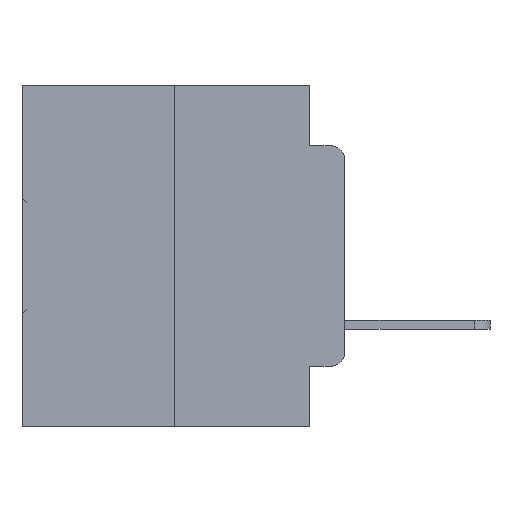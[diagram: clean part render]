
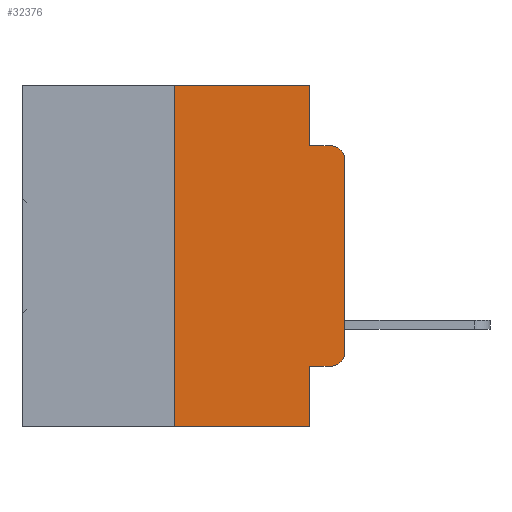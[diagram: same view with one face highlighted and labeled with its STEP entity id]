
A CAD part, left-side view. The second image highlights one B-rep face of the part: STEP entity #32376.
In plain terms, the highlighted planar face has unit normal (-1, 0, 0).
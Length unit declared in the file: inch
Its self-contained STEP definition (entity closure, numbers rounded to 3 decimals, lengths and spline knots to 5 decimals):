
#110 = LINE ( 'NONE', #14499, #1008 ) ;
#382 = ORIENTED_EDGE ( 'NONE', *, *, #10923, .F. ) ;
#1008 = VECTOR ( 'NONE', #17127, 39.37008 ) ;
#1029 = DIRECTION ( 'NONE',  ( 0., -1., 0. ) ) ;
#1550 = CARTESIAN_POINT ( 'NONE',  ( 0., 0.051, 0. ) ) ;
#2625 = EDGE_CURVE ( 'NONE', #13535, #3771, #27099, .T. ) ;
#3015 = ORIENTED_EDGE ( 'NONE', *, *, #16849, .T. ) ;
#3771 = VERTEX_POINT ( 'NONE', #13860 ) ;
#3918 = CIRCLE ( 'NONE', #6936, 0.02 ) ;
#4028 = CARTESIAN_POINT ( 'NONE',  ( 0., 0.051, -0.4115 ) ) ;
#4211 = ORIENTED_EDGE ( 'NONE', *, *, #32056, .T. ) ;
#4632 = CARTESIAN_POINT ( 'NONE',  ( 0., 0.02, -0.3915 ) ) ;
#4680 = VERTEX_POINT ( 'NONE', #14831 ) ;
#5971 = DIRECTION ( 'NONE',  ( 0., 0., 1. ) ) ;
#6571 = CARTESIAN_POINT ( 'NONE',  ( 0., 0.473, 0. ) ) ;
#6590 = VERTEX_POINT ( 'NONE', #17049 ) ;
#6855 = EDGE_CURVE ( 'NONE', #9072, #18997, #19088, .T. ) ;
#6936 = AXIS2_PLACEMENT_3D ( 'NONE', #8356, #26353, #11030 ) ;
#7073 = VERTEX_POINT ( 'NONE', #15179 ) ;
#7368 = DIRECTION ( 'NONE',  ( 0., 0., -1. ) ) ;
#8356 = CARTESIAN_POINT ( 'NONE',  ( 0., 0.02, -0.1085 ) ) ;
#8555 = CARTESIAN_POINT ( 'NONE',  ( 0., 0.25, 0. ) ) ;
#9072 = VERTEX_POINT ( 'NONE', #4028 ) ;
#9272 = DIRECTION ( 'NONE',  ( 0., 0., -1. ) ) ;
#9287 = LINE ( 'NONE', #19518, #15393 ) ;
#10336 = CARTESIAN_POINT ( 'NONE',  ( 0., 0.02, -0.4115 ) ) ;
#10457 = EDGE_CURVE ( 'NONE', #9072, #12935, #26329, .T. ) ;
#10923 = EDGE_CURVE ( 'NONE', #7073, #6590, #9287, .T. ) ;
#10950 = ORIENTED_EDGE ( 'NONE', *, *, #10457, .F. ) ;
#11030 = DIRECTION ( 'NONE',  ( 0., 0., -1. ) ) ;
#11318 = CARTESIAN_POINT ( 'NONE',  ( 0., 0.02, -0.0885 ) ) ;
#11800 = PLANE ( 'NONE',  #18601 ) ;
#12728 = VECTOR ( 'NONE', #21483, 39.37008 ) ;
#12793 = VECTOR ( 'NONE', #22069, 39.37008 ) ;
#12929 = ORIENTED_EDGE ( 'NONE', *, *, #24236, .F. ) ;
#12935 = VERTEX_POINT ( 'NONE', #26229 ) ;
#13535 = VERTEX_POINT ( 'NONE', #28620 ) ;
#13860 = CARTESIAN_POINT ( 'NONE',  ( 0., 0., -0.1085 ) ) ;
#14499 = CARTESIAN_POINT ( 'NONE',  ( 0., 0.051, -0.0885 ) ) ;
#14705 = VERTEX_POINT ( 'NONE', #27469 ) ;
#14831 = CARTESIAN_POINT ( 'NONE',  ( 0., 0.25, -0.5 ) ) ;
#15037 = CIRCLE ( 'NONE', #16231, 0.02 ) ;
#15179 = CARTESIAN_POINT ( 'NONE',  ( 0., 0.25, 0. ) ) ;
#15393 = VECTOR ( 'NONE', #1029, 39.37008 ) ;
#16231 = AXIS2_PLACEMENT_3D ( 'NONE', #4632, #22925, #7368 ) ;
#16281 = CARTESIAN_POINT ( 'NONE',  ( 0., 0.051, -0.4115 ) ) ;
#16462 = DIRECTION ( 'NONE',  ( 0., 0., -1. ) ) ;
#16849 = EDGE_CURVE ( 'NONE', #4680, #12935, #26413, .T. ) ;
#17049 = CARTESIAN_POINT ( 'NONE',  ( 0., 0.051, 0. ) ) ;
#17127 = DIRECTION ( 'NONE',  ( 0., -1., 0. ) ) ;
#17421 = EDGE_CURVE ( 'NONE', #4680, #7073, #21299, .T. ) ;
#17423 = ORIENTED_EDGE ( 'NONE', *, *, #2625, .T. ) ;
#18231 = ORIENTED_EDGE ( 'NONE', *, *, #30620, .F. ) ;
#18601 = AXIS2_PLACEMENT_3D ( 'NONE', #6571, #24701, #9272 ) ;
#18838 = VECTOR ( 'NONE', #27514, 39.37008 ) ;
#18997 = VERTEX_POINT ( 'NONE', #10336 ) ;
#19088 = LINE ( 'NONE', #16281, #25785 ) ;
#19518 = CARTESIAN_POINT ( 'NONE',  ( 0., 0.473, 0. ) ) ;
#19535 = CARTESIAN_POINT ( 'NONE',  ( 0., 0.473, -0.5 ) ) ;
#20516 = VECTOR ( 'NONE', #5971, 39.37008 ) ;
#21299 = LINE ( 'NONE', #8555, #20516 ) ;
#21483 = DIRECTION ( 'NONE',  ( 0., 0., 1. ) ) ;
#22069 = DIRECTION ( 'NONE',  ( 0., -1., 0. ) ) ;
#22751 = VERTEX_POINT ( 'NONE', #11318 ) ;
#22925 = DIRECTION ( 'NONE',  ( -1., 0., 0. ) ) ;
#23002 = ORIENTED_EDGE ( 'NONE', *, *, #17421, .F. ) ;
#23589 = LINE ( 'NONE', #31162, #29303 ) ;
#24236 = EDGE_CURVE ( 'NONE', #6590, #14705, #23589, .T. ) ;
#24701 = DIRECTION ( 'NONE',  ( 1., 0., 0. ) ) ;
#25688 = CARTESIAN_POINT ( 'NONE',  ( 0., 0., 0. ) ) ;
#25785 = VECTOR ( 'NONE', #29824, 39.37008 ) ;
#25835 = FACE_OUTER_BOUND ( 'NONE', #28963, .T. ) ;
#26229 = CARTESIAN_POINT ( 'NONE',  ( 0., 0.051, -0.5 ) ) ;
#26329 = LINE ( 'NONE', #1550, #18838 ) ;
#26353 = DIRECTION ( 'NONE',  ( -1., 0., 0. ) ) ;
#26413 = LINE ( 'NONE', #19535, #12793 ) ;
#27099 = LINE ( 'NONE', #25688, #12728 ) ;
#27469 = CARTESIAN_POINT ( 'NONE',  ( 0., 0.051, -0.0885 ) ) ;
#27514 = DIRECTION ( 'NONE',  ( 0., 0., -1. ) ) ;
#28620 = CARTESIAN_POINT ( 'NONE',  ( 0., 0., -0.3915 ) ) ;
#28963 = EDGE_LOOP ( 'NONE', ( #17423, #4211, #18231, #12929, #382, #23002, #3015, #10950, #30871, #31562 ) ) ;
#29303 = VECTOR ( 'NONE', #16462, 39.37008 ) ;
#29824 = DIRECTION ( 'NONE',  ( 0., -1., 0. ) ) ;
#30620 = EDGE_CURVE ( 'NONE', #14705, #22751, #110, .T. ) ;
#30871 = ORIENTED_EDGE ( 'NONE', *, *, #6855, .T. ) ;
#31162 = CARTESIAN_POINT ( 'NONE',  ( 0., 0.051, 0. ) ) ;
#31562 = ORIENTED_EDGE ( 'NONE', *, *, #32594, .T. ) ;
#32056 = EDGE_CURVE ( 'NONE', #3771, #22751, #3918, .T. ) ;
#32376 = ADVANCED_FACE ( 'NONE', ( #25835 ), #11800, .F. ) ;
#32594 = EDGE_CURVE ( 'NONE', #18997, #13535, #15037, .T. ) ;
